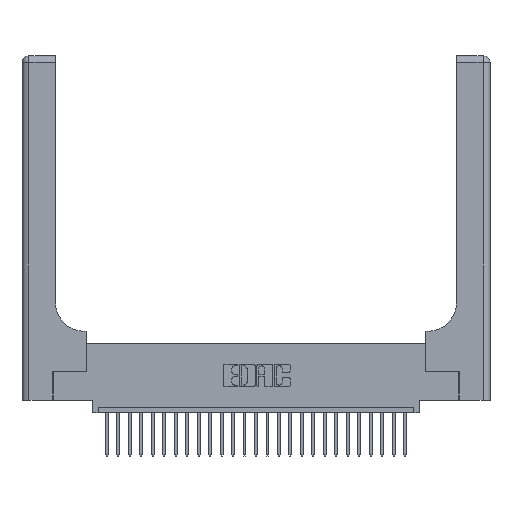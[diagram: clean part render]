
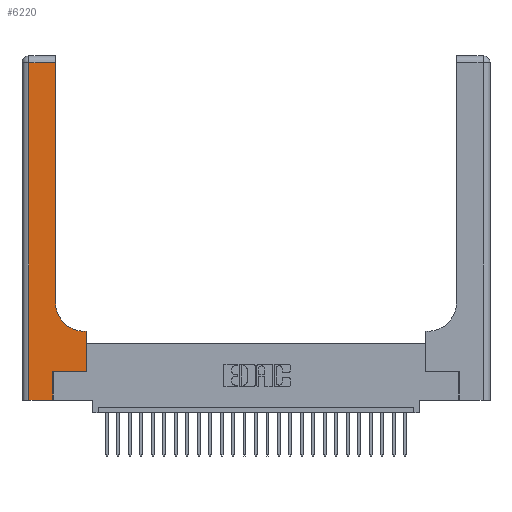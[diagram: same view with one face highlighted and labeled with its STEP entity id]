
A CAD part, top view. The second image highlights one B-rep face of the part: STEP entity #6220.
In plain terms, the highlighted planar face has unit normal (0, 0, 1).
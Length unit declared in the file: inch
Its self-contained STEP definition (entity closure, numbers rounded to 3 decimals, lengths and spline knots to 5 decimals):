
#64 = VECTOR ( 'NONE', #6806, 39.37008 ) ;
#147 = VERTEX_POINT ( 'NONE', #23745 ) ;
#816 = DIRECTION ( 'NONE',  ( 0., 1., 0. ) ) ;
#946 = VERTEX_POINT ( 'NONE', #15754 ) ;
#954 = ORIENTED_EDGE ( 'NONE', *, *, #16112, .T. ) ;
#1083 = EDGE_CURVE ( 'NONE', #946, #5331, #9794, .T. ) ;
#1159 = LINE ( 'NONE', #21108, #2491 ) ;
#1488 = DIRECTION ( 'NONE',  ( -1., 0., 0. ) ) ;
#1551 = ORIENTED_EDGE ( 'NONE', *, *, #24186, .T. ) ;
#2177 = EDGE_CURVE ( 'NONE', #2984, #26470, #16747, .T. ) ;
#2302 = DIRECTION ( 'NONE',  ( 1., 0., 0. ) ) ;
#2491 = VECTOR ( 'NONE', #18589, 39.37008 ) ;
#2984 = VERTEX_POINT ( 'NONE', #5577 ) ;
#3221 = LINE ( 'NONE', #24267, #26280 ) ;
#3246 = ORIENTED_EDGE ( 'NONE', *, *, #9990, .T. ) ;
#3378 = CARTESIAN_POINT ( 'NONE',  ( 0.06, 2.94, 0.37 ) ) ;
#3640 = DIRECTION ( 'NONE',  ( 0., 1., 0. ) ) ;
#3921 = VECTOR ( 'NONE', #2302, 39.37008 ) ;
#4938 = PLANE ( 'NONE',  #11374 ) ;
#5023 = DIRECTION ( 'NONE',  ( -1., 0., 0. ) ) ;
#5155 = LINE ( 'NONE', #5962, #9536 ) ;
#5331 = VERTEX_POINT ( 'NONE', #3378 ) ;
#5577 = CARTESIAN_POINT ( 'NONE',  ( 0.5585, 0.6, 0.37 ) ) ;
#5723 = VERTEX_POINT ( 'NONE', #7278 ) ;
#5832 = EDGE_CURVE ( 'NONE', #22827, #946, #5155, .T. ) ;
#5962 = CARTESIAN_POINT ( 'NONE',  ( 0.2915, 3., 0.37 ) ) ;
#6220 = ADVANCED_FACE ( 'NONE', ( #8025 ), #4938, .F. ) ;
#6404 = CARTESIAN_POINT ( 'NONE',  ( 0.5415, 0.85, 0.37 ) ) ;
#6579 = ORIENTED_EDGE ( 'NONE', *, *, #1083, .T. ) ;
#6806 = DIRECTION ( 'NONE',  ( -1., 0., 0. ) ) ;
#7278 = CARTESIAN_POINT ( 'NONE',  ( 0.06, 0., 0.37 ) ) ;
#7795 = CARTESIAN_POINT ( 'NONE',  ( 0.5585, 0.25, 0.37 ) ) ;
#8025 = FACE_OUTER_BOUND ( 'NONE', #24124, .T. ) ;
#9323 = ORIENTED_EDGE ( 'NONE', *, *, #5832, .T. ) ;
#9536 = VECTOR ( 'NONE', #14600, 39.37008 ) ;
#9794 = LINE ( 'NONE', #19634, #64 ) ;
#9990 = EDGE_CURVE ( 'NONE', #147, #14183, #25834, .T. ) ;
#10307 = CIRCLE ( 'NONE', #27275, 0.25 ) ;
#11374 = AXIS2_PLACEMENT_3D ( 'NONE', #17843, #22059, #5023 ) ;
#12222 = ORIENTED_EDGE ( 'NONE', *, *, #26524, .T. ) ;
#12788 = ORIENTED_EDGE ( 'NONE', *, *, #16482, .T. ) ;
#14183 = VERTEX_POINT ( 'NONE', #24729 ) ;
#14289 = LINE ( 'NONE', #27014, #19284 ) ;
#14600 = DIRECTION ( 'NONE',  ( 0., 1., 0. ) ) ;
#14746 = VECTOR ( 'NONE', #1488, 39.37008 ) ;
#15754 = CARTESIAN_POINT ( 'NONE',  ( 0.2915, 2.94, 0.37 ) ) ;
#15795 = VERTEX_POINT ( 'NONE', #7795 ) ;
#16112 = EDGE_CURVE ( 'NONE', #15795, #2984, #3221, .T. ) ;
#16482 = EDGE_CURVE ( 'NONE', #26470, #22827, #10307, .T. ) ;
#16747 = LINE ( 'NONE', #27097, #14746 ) ;
#17843 = CARTESIAN_POINT ( 'NONE',  ( 0., 3., 0.37 ) ) ;
#18288 = LINE ( 'NONE', #26098, #3921 ) ;
#18589 = DIRECTION ( 'NONE',  ( 0., -1., 0. ) ) ;
#18633 = DIRECTION ( 'NONE',  ( 1., 0., 0. ) ) ;
#19201 = VECTOR ( 'NONE', #3640, 39.37008 ) ;
#19284 = VECTOR ( 'NONE', #22915, 39.37008 ) ;
#19634 = CARTESIAN_POINT ( 'NONE',  ( 0., 2.94, 0.37 ) ) ;
#20769 = CARTESIAN_POINT ( 'NONE',  ( 0.5415, 0.6, 0.37 ) ) ;
#21108 = CARTESIAN_POINT ( 'NONE',  ( 0.06, 3., 0.37 ) ) ;
#22059 = DIRECTION ( 'NONE',  ( 0., 0., -1. ) ) ;
#22764 = CARTESIAN_POINT ( 'NONE',  ( 0.2915, 0.85, 0.37 ) ) ;
#22827 = VERTEX_POINT ( 'NONE', #22764 ) ;
#22915 = DIRECTION ( 'NONE',  ( 1., 0., 0. ) ) ;
#23106 = ORIENTED_EDGE ( 'NONE', *, *, #2177, .T. ) ;
#23745 = CARTESIAN_POINT ( 'NONE',  ( 0.269, 0., 0.37 ) ) ;
#24124 = EDGE_LOOP ( 'NONE', ( #9323, #6579, #25234, #12222, #3246, #1551, #954, #23106, #12788 ) ) ;
#24186 = EDGE_CURVE ( 'NONE', #14183, #15795, #18288, .T. ) ;
#24267 = CARTESIAN_POINT ( 'NONE',  ( 0.5585, 0.25, 0.37 ) ) ;
#24729 = CARTESIAN_POINT ( 'NONE',  ( 0.269, 0.25, 0.37 ) ) ;
#24949 = CARTESIAN_POINT ( 'NONE',  ( 0.269, 0., 0.37 ) ) ;
#25234 = ORIENTED_EDGE ( 'NONE', *, *, #27244, .T. ) ;
#25663 = DIRECTION ( 'NONE',  ( 0., 0., -1. ) ) ;
#25834 = LINE ( 'NONE', #24949, #19201 ) ;
#26098 = CARTESIAN_POINT ( 'NONE',  ( 0.269, 0.25, 0.37 ) ) ;
#26280 = VECTOR ( 'NONE', #816, 39.37008 ) ;
#26470 = VERTEX_POINT ( 'NONE', #20769 ) ;
#26524 = EDGE_CURVE ( 'NONE', #5723, #147, #14289, .T. ) ;
#27014 = CARTESIAN_POINT ( 'NONE',  ( 0., 0., 0.37 ) ) ;
#27097 = CARTESIAN_POINT ( 'NONE',  ( 0.2915, 0.6, 0.37 ) ) ;
#27244 = EDGE_CURVE ( 'NONE', #5331, #5723, #1159, .T. ) ;
#27275 = AXIS2_PLACEMENT_3D ( 'NONE', #6404, #25663, #18633 ) ;
